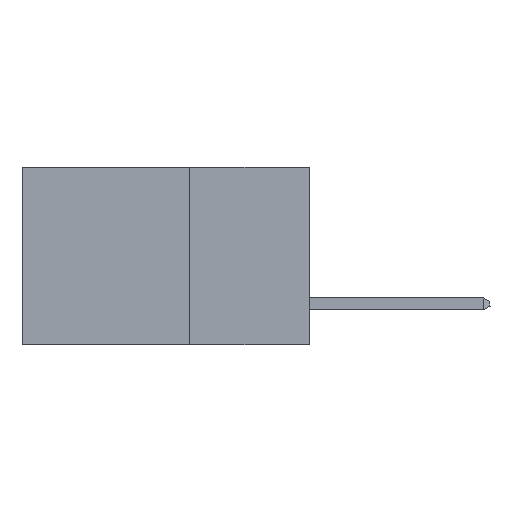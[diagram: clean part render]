
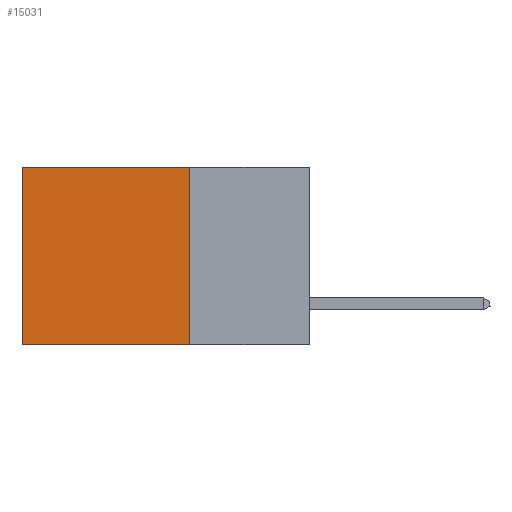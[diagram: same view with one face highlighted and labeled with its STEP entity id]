
A CAD part, left-side view. The second image highlights one B-rep face of the part: STEP entity #15031.
In plain terms, the highlighted planar face has unit normal (-1, 0, 0).
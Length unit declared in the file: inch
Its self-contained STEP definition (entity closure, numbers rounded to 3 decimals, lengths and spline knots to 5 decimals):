
#811 = CARTESIAN_POINT ( 'NONE',  ( 0.2875, 0.25, 0. ) ) ;
#1191 = DIRECTION ( 'NONE',  ( 1., 0., 0. ) ) ;
#2260 = CARTESIAN_POINT ( 'NONE',  ( 0.2875, 0.25, -0.37 ) ) ;
#2583 = ORIENTED_EDGE ( 'NONE', *, *, #14646, .T. ) ;
#3519 = LINE ( 'NONE', #26155, #17611 ) ;
#7244 = CARTESIAN_POINT ( 'NONE',  ( 0.2875, 0.6, 0. ) ) ;
#7311 = CARTESIAN_POINT ( 'NONE',  ( 0.2875, 0.6, 0. ) ) ;
#8494 = VERTEX_POINT ( 'NONE', #7244 ) ;
#9040 = PLANE ( 'NONE',  #21814 ) ;
#10226 = DIRECTION ( 'NONE',  ( 0., 1., 0. ) ) ;
#11718 = VERTEX_POINT ( 'NONE', #22241 ) ;
#11934 = ORIENTED_EDGE ( 'NONE', *, *, #20579, .T. ) ;
#12453 = LINE ( 'NONE', #2260, #31819 ) ;
#13943 = LINE ( 'NONE', #7311, #25567 ) ;
#14355 = CARTESIAN_POINT ( 'NONE',  ( 0.2875, 0.25, 0. ) ) ;
#14458 = CARTESIAN_POINT ( 'NONE',  ( 0.2875, 0.25, -0.37 ) ) ;
#14646 = EDGE_CURVE ( 'NONE', #24994, #8494, #3519, .T. ) ;
#15031 = ADVANCED_FACE ( 'NONE', ( #26329 ), #9040, .F. ) ;
#17043 = CARTESIAN_POINT ( 'NONE',  ( 0.2875, 0.25, 0. ) ) ;
#17611 = VECTOR ( 'NONE', #10226, 39.37008 ) ;
#17870 = VECTOR ( 'NONE', #22036, 39.37008 ) ;
#19724 = DIRECTION ( 'NONE',  ( 0., 0., -1. ) ) ;
#20579 = EDGE_CURVE ( 'NONE', #8494, #11718, #13943, .T. ) ;
#21814 = AXIS2_PLACEMENT_3D ( 'NONE', #17043, #1191, #19724 ) ;
#22036 = DIRECTION ( 'NONE',  ( 0., 0., -1. ) ) ;
#22216 = ORIENTED_EDGE ( 'NONE', *, *, #34005, .F. ) ;
#22241 = CARTESIAN_POINT ( 'NONE',  ( 0.2875, 0.6, -0.37 ) ) ;
#22716 = ORIENTED_EDGE ( 'NONE', *, *, #23676, .F. ) ;
#23249 = DIRECTION ( 'NONE',  ( 0., 0., -1. ) ) ;
#23676 = EDGE_CURVE ( 'NONE', #24994, #30643, #24977, .T. ) ;
#23783 = EDGE_LOOP ( 'NONE', ( #11934, #22216, #22716, #2583 ) ) ;
#24977 = LINE ( 'NONE', #811, #17870 ) ;
#24994 = VERTEX_POINT ( 'NONE', #14355 ) ;
#25567 = VECTOR ( 'NONE', #23249, 39.37008 ) ;
#26155 = CARTESIAN_POINT ( 'NONE',  ( 0.2875, 0.25, 0. ) ) ;
#26329 = FACE_OUTER_BOUND ( 'NONE', #23783, .T. ) ;
#30643 = VERTEX_POINT ( 'NONE', #14458 ) ;
#30837 = DIRECTION ( 'NONE',  ( 0., 1., 0. ) ) ;
#31819 = VECTOR ( 'NONE', #30837, 39.37008 ) ;
#34005 = EDGE_CURVE ( 'NONE', #30643, #11718, #12453, .T. ) ;
